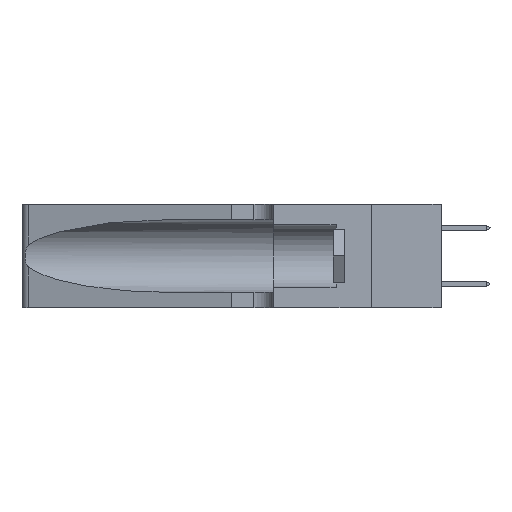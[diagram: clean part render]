
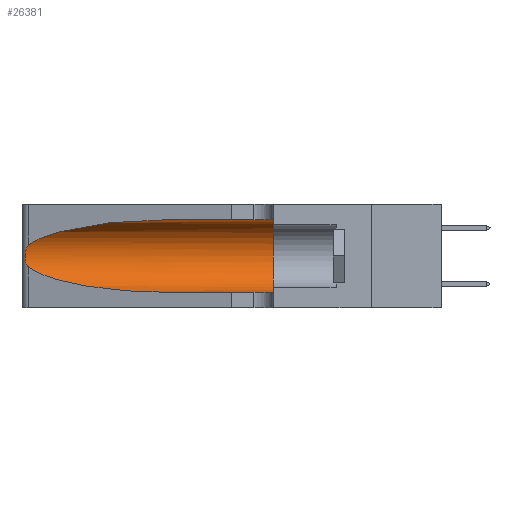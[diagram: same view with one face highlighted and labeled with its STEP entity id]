
A CAD part, left-side view. The second image highlights one B-rep face of the part: STEP entity #26381.
In plain terms, the highlighted cylindrical face has radius 3.308 mm (diameter 6.617 mm), a partial arc.
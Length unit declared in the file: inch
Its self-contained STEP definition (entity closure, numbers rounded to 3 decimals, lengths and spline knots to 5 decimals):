
#203 = VERTEX_POINT ( 'NONE', #38835 ) ;
#975 = CARTESIAN_POINT ( 'NONE',  ( 0.1305, 0.35, 0.185 ) ) ;
#2183 = CARTESIAN_POINT ( 'NONE',  ( 0.18966, 0.96281, 0.31525 ) ) ;
#2339 = CARTESIAN_POINT ( 'NONE',  ( 0.25487, 1.22718, 0.14631 ) ) ;
#2886 = CARTESIAN_POINT ( 'NONE',  ( 0.26017, 1.23833, 0.17102 ) ) ;
#3724 = DIRECTION ( 'NONE',  ( 0., -1., 0. ) ) ;
#3904 = ORIENTED_EDGE ( 'NONE', *, *, #12679, .F. ) ;
#5357 = CARTESIAN_POINT ( 'NONE',  ( 0.1305, 0.35, 0.31525 ) ) ;
#6973 = DIRECTION ( 'NONE',  ( 0., 0., 1. ) ) ;
#8194 = VERTEX_POINT ( 'NONE', #5357 ) ;
#9609 = CARTESIAN_POINT ( 'NONE',  ( 0.25789, 1.23486, 0.15765 ) ) ;
#10849 = VERTEX_POINT ( 'NONE', #19611 ) ;
#11005 = B_SPLINE_CURVE_WITH_KNOTS ( 'NONE', 3,
 ( #28952, #15625, #32690, #16184, #29506, #19501, #22863, #12373, #2886, #25773, #9609, #18936, #15906, #35625 ),
 .UNSPECIFIED., .F., .F.,
 ( 4, 2, 2, 2, 2, 2, 4 ),
 ( 0., 0.00027, 0.00053, 0.00107, 0.0016, 0.00187, 0.00214 ),
 .UNSPECIFIED. ) ;
#11129 = AXIS2_PLACEMENT_3D ( 'NONE', #975, #37185, #6973 ) ;
#11780 = DIRECTION ( 'NONE',  ( 0., 0., -1. ) ) ;
#12373 = CARTESIAN_POINT ( 'NONE',  ( 0.26075, 1.23896, 0.178 ) ) ;
#12679 = EDGE_CURVE ( 'NONE', #8194, #25964, #32735, .T. ) ;
#13864 = VECTOR ( 'NONE', #3724, 39.37008 ) ;
#15625 = CARTESIAN_POINT ( 'NONE',  ( 0.25555, 1.22994, 0.2215 ) ) ;
#15906 = CARTESIAN_POINT ( 'NONE',  ( 0.25555, 1.22993, 0.14849 ) ) ;
#16184 = CARTESIAN_POINT ( 'NONE',  ( 0.25787, 1.23484, 0.2124 ) ) ;
#17284 = EDGE_CURVE ( 'NONE', #32650, #25964, #24227, .T. ) ;
#18454 = CARTESIAN_POINT ( 'NONE',  ( 0.1305, 0.35, 0.05475 ) ) ;
#18917 = EDGE_CURVE ( 'NONE', #42035, #10849, #20593, .T. ) ;
#18936 = CARTESIAN_POINT ( 'NONE',  ( 0.25639, 1.23186, 0.15144 ) ) ;
#19080 = CARTESIAN_POINT ( 'NONE',  ( 0.25487, 1.22718, 0.22369 ) ) ;
#19120 = LINE ( 'NONE', #37313, #13864 ) ;
#19501 = CARTESIAN_POINT ( 'NONE',  ( 0.26018, 1.23835, 0.19895 ) ) ;
#19611 = CARTESIAN_POINT ( 'NONE',  ( 0.25487, 1.22718, 0.22369 ) ) ;
#20156 = DIRECTION ( 'NONE',  ( 0., -1., 0. ) ) ;
#20593 =( BOUNDED_CURVE ( )  B_SPLINE_CURVE ( 3, ( #35169, #2183, #32134, #19080 ),
 .UNSPECIFIED., .F., .F. ) 
 B_SPLINE_CURVE_WITH_KNOTS ( ( 4, 4 ),
 ( 1.5708, 2.84003 ),
 .UNSPECIFIED. ) 
 CURVE ( )  GEOMETRIC_REPRESENTATION_ITEM ( )  RATIONAL_B_SPLINE_CURVE ( ( 1., 0.87, 0.87, 1. ) ) 
 REPRESENTATION_ITEM ( '' )  );
#20644 = ORIENTED_EDGE ( 'NONE', *, *, #33322, .F. ) ;
#21817 = AXIS2_PLACEMENT_3D ( 'NONE', #34402, #34853, #11780 ) ;
#21987 = EDGE_CURVE ( 'NONE', #10849, #203, #11005, .T. ) ;
#22863 = CARTESIAN_POINT ( 'NONE',  ( 0.26075, 1.23896, 0.19203 ) ) ;
#24227 = LINE ( 'NONE', #42092, #27322 ) ;
#24671 = ORIENTED_EDGE ( 'NONE', *, *, #41835, .T. ) ;
#25773 = CARTESIAN_POINT ( 'NONE',  ( 0.25856, 1.23593, 0.16098 ) ) ;
#25964 = VERTEX_POINT ( 'NONE', #18454 ) ;
#26321 = ORIENTED_EDGE ( 'NONE', *, *, #21987, .T. ) ;
#26381 = ADVANCED_FACE ( 'NONE', ( #41955 ), #36717, .F. ) ;
#26683 = EDGE_LOOP ( 'NONE', ( #27207, #26321, #24671, #40610, #3904, #20644 ) ) ;
#27207 = ORIENTED_EDGE ( 'NONE', *, *, #18917, .T. ) ;
#27322 = VECTOR ( 'NONE', #20156, 39.37008 ) ;
#28952 = CARTESIAN_POINT ( 'NONE',  ( 0.25487, 1.22718, 0.22369 ) ) ;
#29125 = CARTESIAN_POINT ( 'NONE',  ( 0.2373, 1.15595, 0.08982 ) ) ;
#29506 = CARTESIAN_POINT ( 'NONE',  ( 0.25854, 1.2359, 0.20912 ) ) ;
#29806 = CARTESIAN_POINT ( 'NONE',  ( 0.1305, 0.72297, 0.31525 ) ) ;
#32134 = CARTESIAN_POINT ( 'NONE',  ( 0.2373, 1.15595, 0.28018 ) ) ;
#32650 = VERTEX_POINT ( 'NONE', #41373 ) ;
#32690 = CARTESIAN_POINT ( 'NONE',  ( 0.25639, 1.23184, 0.21858 ) ) ;
#32735 = CIRCLE ( 'NONE', #11129, 0.13025 ) ;
#33322 = EDGE_CURVE ( 'NONE', #42035, #8194, #19120, .T. ) ;
#34402 = CARTESIAN_POINT ( 'NONE',  ( 0.1305, 1.61858, 0.185 ) ) ;
#34853 = DIRECTION ( 'NONE',  ( 0., -1., 0. ) ) ;
#35169 = CARTESIAN_POINT ( 'NONE',  ( 0.1305, 0.72297, 0.31525 ) ) ;
#35625 = CARTESIAN_POINT ( 'NONE',  ( 0.25487, 1.22718, 0.14631 ) ) ;
#35648 = CARTESIAN_POINT ( 'NONE',  ( 0.18966, 0.96281, 0.05475 ) ) ;
#35929 = CARTESIAN_POINT ( 'NONE',  ( 0.1305, 0.72297, 0.05475 ) ) ;
#36717 = CYLINDRICAL_SURFACE ( 'NONE', #21817, 0.13025 ) ;
#37185 = DIRECTION ( 'NONE',  ( 0., 1., 0. ) ) ;
#37313 = CARTESIAN_POINT ( 'NONE',  ( 0.1305, 1.61858, 0.31525 ) ) ;
#38835 = CARTESIAN_POINT ( 'NONE',  ( 0.25487, 1.22718, 0.14631 ) ) ;
#40610 = ORIENTED_EDGE ( 'NONE', *, *, #17284, .T. ) ;
#41373 = CARTESIAN_POINT ( 'NONE',  ( 0.1305, 0.72297, 0.05475 ) ) ;
#41835 = EDGE_CURVE ( 'NONE', #203, #32650, #42503, .T. ) ;
#41955 = FACE_OUTER_BOUND ( 'NONE', #26683, .T. ) ;
#42035 = VERTEX_POINT ( 'NONE', #29806 ) ;
#42092 = CARTESIAN_POINT ( 'NONE',  ( 0.1305, 1.61858, 0.05475 ) ) ;
#42503 =( BOUNDED_CURVE ( )  B_SPLINE_CURVE ( 3, ( #2339, #29125, #35648, #35929 ),
 .UNSPECIFIED., .F., .F. ) 
 B_SPLINE_CURVE_WITH_KNOTS ( ( 4, 4 ),
 ( 3.44316, 4.71239 ),
 .UNSPECIFIED. ) 
 CURVE ( )  GEOMETRIC_REPRESENTATION_ITEM ( )  RATIONAL_B_SPLINE_CURVE ( ( 1., 0.87, 0.87, 1. ) ) 
 REPRESENTATION_ITEM ( '' )  );
